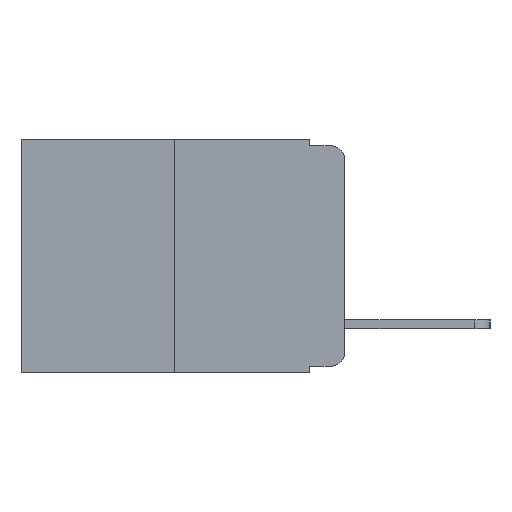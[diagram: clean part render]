
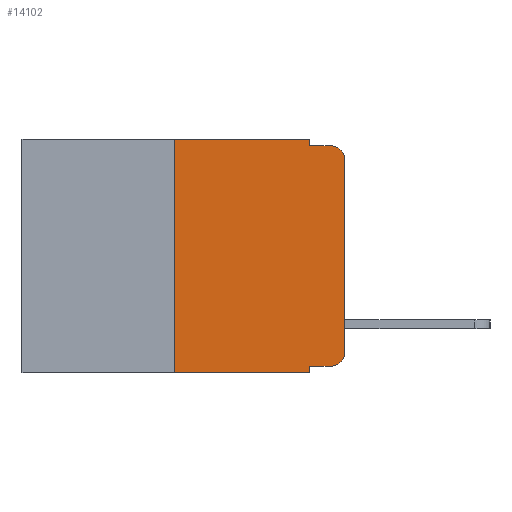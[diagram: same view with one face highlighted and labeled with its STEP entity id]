
A CAD part, left-side view. The second image highlights one B-rep face of the part: STEP entity #14102.
In plain terms, the highlighted planar face has unit normal (-1, 0, 0).
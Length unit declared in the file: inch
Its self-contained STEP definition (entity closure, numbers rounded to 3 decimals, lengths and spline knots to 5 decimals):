
#382 = VERTEX_POINT ( 'NONE', #15111 ) ;
#591 = CARTESIAN_POINT ( 'NONE',  ( 0., 0.473, -0.343 ) ) ;
#657 = EDGE_CURVE ( 'NONE', #18046, #12614, #15552, .T. ) ;
#1487 = CARTESIAN_POINT ( 'NONE',  ( 0., 0.051, -0.01 ) ) ;
#1735 = EDGE_CURVE ( 'NONE', #12614, #382, #16211, .T. ) ;
#2316 = CARTESIAN_POINT ( 'NONE',  ( 0., 0.02, -0.03 ) ) ;
#2361 = VECTOR ( 'NONE', #7938, 39.37008 ) ;
#2815 = EDGE_CURVE ( 'NONE', #4068, #382, #15454, .T. ) ;
#3045 = ORIENTED_EDGE ( 'NONE', *, *, #19988, .F. ) ;
#3193 = PLANE ( 'NONE',  #19819 ) ;
#3293 = DIRECTION ( 'NONE',  ( 0., 0., 1. ) ) ;
#3544 = ORIENTED_EDGE ( 'NONE', *, *, #18991, .F. ) ;
#3897 = EDGE_CURVE ( 'NONE', #17990, #4068, #12040, .T. ) ;
#3957 = DIRECTION ( 'NONE',  ( 0., 0., -1. ) ) ;
#4049 = ORIENTED_EDGE ( 'NONE', *, *, #17982, .T. ) ;
#4068 = VERTEX_POINT ( 'NONE', #12875 ) ;
#5252 = DIRECTION ( 'NONE',  ( -1., 0., 0. ) ) ;
#6000 = CARTESIAN_POINT ( 'NONE',  ( 0., 0., 0. ) ) ;
#6326 = VECTOR ( 'NONE', #13377, 39.37008 ) ;
#6453 = DIRECTION ( 'NONE',  ( 1., 0., 0. ) ) ;
#6654 = VERTEX_POINT ( 'NONE', #9982 ) ;
#6732 = EDGE_CURVE ( 'NONE', #17329, #12542, #14701, .T. ) ;
#6825 = ORIENTED_EDGE ( 'NONE', *, *, #657, .F. ) ;
#7183 = VECTOR ( 'NONE', #3957, 39.37008 ) ;
#7302 = VECTOR ( 'NONE', #15443, 39.37008 ) ;
#7938 = DIRECTION ( 'NONE',  ( 0., -1., 0. ) ) ;
#8054 = DIRECTION ( 'NONE',  ( 0., -1., 0. ) ) ;
#9084 = VERTEX_POINT ( 'NONE', #9543 ) ;
#9543 = CARTESIAN_POINT ( 'NONE',  ( 0., 0.25, 0. ) ) ;
#9822 = LINE ( 'NONE', #15412, #17605 ) ;
#9982 = CARTESIAN_POINT ( 'NONE',  ( 0., 0.051, -0.333 ) ) ;
#10371 = CARTESIAN_POINT ( 'NONE',  ( 0., 0.473, 0. ) ) ;
#10531 = VECTOR ( 'NONE', #3293, 39.37008 ) ;
#10546 = AXIS2_PLACEMENT_3D ( 'NONE', #2316, #13486, #17193 ) ;
#11016 = LINE ( 'NONE', #11266, #10531 ) ;
#11055 = ORIENTED_EDGE ( 'NONE', *, *, #18878, .F. ) ;
#11131 = AXIS2_PLACEMENT_3D ( 'NONE', #14722, #5252, #16275 ) ;
#11266 = CARTESIAN_POINT ( 'NONE',  ( 0., 0.25, 0. ) ) ;
#11556 = ORIENTED_EDGE ( 'NONE', *, *, #6732, .T. ) ;
#11965 = DIRECTION ( 'NONE',  ( 0., -1., 0. ) ) ;
#12040 = LINE ( 'NONE', #6000, #7302 ) ;
#12120 = VECTOR ( 'NONE', #8054, 39.37008 ) ;
#12498 = CARTESIAN_POINT ( 'NONE',  ( 0., 0.25, -0.343 ) ) ;
#12542 = VERTEX_POINT ( 'NONE', #18124 ) ;
#12553 = ORIENTED_EDGE ( 'NONE', *, *, #16980, .T. ) ;
#12614 = VERTEX_POINT ( 'NONE', #16785 ) ;
#12687 = CARTESIAN_POINT ( 'NONE',  ( 0., 0.051, -0.333 ) ) ;
#12875 = CARTESIAN_POINT ( 'NONE',  ( 0., 0., -0.03 ) ) ;
#13049 = CIRCLE ( 'NONE', #11131, 0.02 ) ;
#13310 = CARTESIAN_POINT ( 'NONE',  ( 0., 0.051, 0. ) ) ;
#13377 = DIRECTION ( 'NONE',  ( 0., -1., 0. ) ) ;
#13486 = DIRECTION ( 'NONE',  ( -1., 0., 0. ) ) ;
#14102 = ADVANCED_FACE ( 'NONE', ( #18862 ), #3193, .F. ) ;
#14701 = LINE ( 'NONE', #591, #6326 ) ;
#14705 = ORIENTED_EDGE ( 'NONE', *, *, #1735, .F. ) ;
#14722 = CARTESIAN_POINT ( 'NONE',  ( 0., 0.02, -0.313 ) ) ;
#14859 = CARTESIAN_POINT ( 'NONE',  ( 0., 0.02, -0.333 ) ) ;
#15111 = CARTESIAN_POINT ( 'NONE',  ( 0., 0.02, -0.01 ) ) ;
#15172 = EDGE_LOOP ( 'NONE', ( #17347, #18308, #14705, #6825, #11055, #3045, #11556, #3544, #4049, #12553 ) ) ;
#15412 = CARTESIAN_POINT ( 'NONE',  ( 0., 0.051, 0. ) ) ;
#15443 = DIRECTION ( 'NONE',  ( 0., 0., 1. ) ) ;
#15454 = CIRCLE ( 'NONE', #10546, 0.02 ) ;
#15552 = LINE ( 'NONE', #13310, #7183 ) ;
#15845 = CARTESIAN_POINT ( 'NONE',  ( 0., 0.473, 0. ) ) ;
#16211 = LINE ( 'NONE', #1487, #12120 ) ;
#16275 = DIRECTION ( 'NONE',  ( 0., 0., -1. ) ) ;
#16785 = CARTESIAN_POINT ( 'NONE',  ( 0., 0.051, -0.01 ) ) ;
#16911 = LINE ( 'NONE', #10371, #20397 ) ;
#16962 = DIRECTION ( 'NONE',  ( 0., 0., -1. ) ) ;
#16980 = EDGE_CURVE ( 'NONE', #17064, #17990, #13049, .T. ) ;
#17064 = VERTEX_POINT ( 'NONE', #14859 ) ;
#17193 = DIRECTION ( 'NONE',  ( 0., 0., -1. ) ) ;
#17307 = CARTESIAN_POINT ( 'NONE',  ( 0., 0., -0.313 ) ) ;
#17329 = VERTEX_POINT ( 'NONE', #12498 ) ;
#17347 = ORIENTED_EDGE ( 'NONE', *, *, #3897, .T. ) ;
#17390 = DIRECTION ( 'NONE',  ( 0., 0., -1. ) ) ;
#17445 = CARTESIAN_POINT ( 'NONE',  ( 0., 0.051, 0. ) ) ;
#17605 = VECTOR ( 'NONE', #16962, 39.37008 ) ;
#17982 = EDGE_CURVE ( 'NONE', #6654, #17064, #18618, .T. ) ;
#17990 = VERTEX_POINT ( 'NONE', #17307 ) ;
#18046 = VERTEX_POINT ( 'NONE', #17445 ) ;
#18124 = CARTESIAN_POINT ( 'NONE',  ( 0., 0.051, -0.343 ) ) ;
#18308 = ORIENTED_EDGE ( 'NONE', *, *, #2815, .T. ) ;
#18618 = LINE ( 'NONE', #12687, #2361 ) ;
#18862 = FACE_OUTER_BOUND ( 'NONE', #15172, .T. ) ;
#18878 = EDGE_CURVE ( 'NONE', #9084, #18046, #16911, .T. ) ;
#18991 = EDGE_CURVE ( 'NONE', #6654, #12542, #9822, .T. ) ;
#19819 = AXIS2_PLACEMENT_3D ( 'NONE', #15845, #6453, #17390 ) ;
#19988 = EDGE_CURVE ( 'NONE', #17329, #9084, #11016, .T. ) ;
#20397 = VECTOR ( 'NONE', #11965, 39.37008 ) ;
